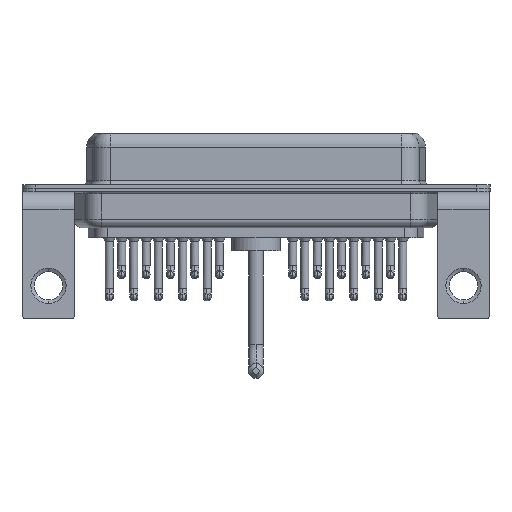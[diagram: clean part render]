
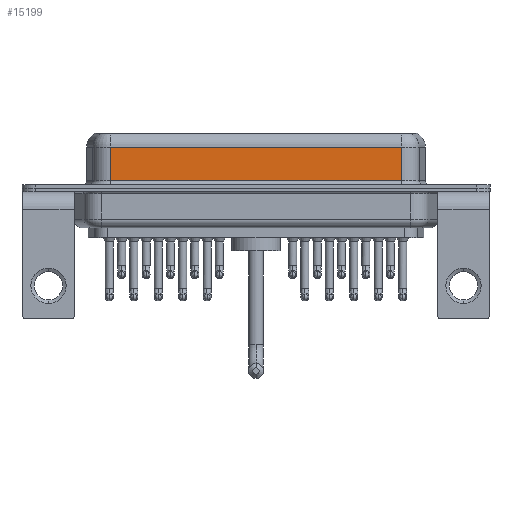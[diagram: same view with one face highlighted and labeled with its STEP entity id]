
A CAD part, front view. The second image highlights one B-rep face of the part: STEP entity #15199.
In plain terms, the highlighted planar face has unit normal (0, -1, 0).
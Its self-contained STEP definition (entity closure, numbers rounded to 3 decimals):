
#224 = DIRECTION ( 'NONE',  ( 0., 0., -1. ) ) ;
#295 = EDGE_LOOP ( 'NONE', ( #20281, #18069, #9514, #14334 ) ) ;
#2162 = CARTESIAN_POINT ( 'NONE',  ( 40.037, -3.95, 6.4 ) ) ;
#2310 = CARTESIAN_POINT ( 'NONE',  ( 40.037, -3.95, 4.65 ) ) ;
#2515 = CARTESIAN_POINT ( 'NONE',  ( 40.037, -3.95, 4.65 ) ) ;
#3378 = VECTOR ( 'NONE', #14742, 1000. ) ;
#3466 = VERTEX_POINT ( 'NONE', #2515 ) ;
#3902 = CARTESIAN_POINT ( 'NONE',  ( 7.013, -3.95, 6.4 ) ) ;
#4205 = CARTESIAN_POINT ( 'NONE',  ( 7.013, -3.95, 0.9 ) ) ;
#5093 = VECTOR ( 'NONE', #5467, 1000. ) ;
#5361 = VECTOR ( 'NONE', #8399, 1000. ) ;
#5467 = DIRECTION ( 'NONE',  ( 0., 0., -1. ) ) ;
#5949 = FACE_OUTER_BOUND ( 'NONE', #295, .T. ) ;
#6619 = CARTESIAN_POINT ( 'NONE',  ( 40.037, -3.95, 0.9 ) ) ;
#7416 = LINE ( 'NONE', #2310, #3378 ) ;
#7701 = VERTEX_POINT ( 'NONE', #11020 ) ;
#8399 = DIRECTION ( 'NONE',  ( 1., 0., 0. ) ) ;
#8780 = LINE ( 'NONE', #14222, #11009 ) ;
#9302 = EDGE_CURVE ( 'NONE', #3466, #20092, #7416, .T. ) ;
#9390 = DIRECTION ( 'NONE',  ( 0., 1., 0. ) ) ;
#9514 = ORIENTED_EDGE ( 'NONE', *, *, #11217, .T. ) ;
#11009 = VECTOR ( 'NONE', #224, 1000. ) ;
#11020 = CARTESIAN_POINT ( 'NONE',  ( 40.037, -3.95, 0.9 ) ) ;
#11175 = DIRECTION ( 'NONE',  ( 0., 0., 1. ) ) ;
#11217 = EDGE_CURVE ( 'NONE', #20092, #21561, #12791, .T. ) ;
#12791 = LINE ( 'NONE', #3902, #5093 ) ;
#13318 = AXIS2_PLACEMENT_3D ( 'NONE', #2162, #9390, #11175 ) ;
#14222 = CARTESIAN_POINT ( 'NONE',  ( 40.037, -3.95, 6.4 ) ) ;
#14334 = ORIENTED_EDGE ( 'NONE', *, *, #19742, .T. ) ;
#14742 = DIRECTION ( 'NONE',  ( -1., 0., 0. ) ) ;
#14987 = CARTESIAN_POINT ( 'NONE',  ( 7.013, -3.95, 4.65 ) ) ;
#15199 = ADVANCED_FACE ( 'NONE', ( #5949 ), #20360, .F. ) ;
#17370 = LINE ( 'NONE', #6619, #5361 ) ;
#18069 = ORIENTED_EDGE ( 'NONE', *, *, #9302, .T. ) ;
#19454 = EDGE_CURVE ( 'NONE', #3466, #7701, #8780, .T. ) ;
#19742 = EDGE_CURVE ( 'NONE', #21561, #7701, #17370, .T. ) ;
#20092 = VERTEX_POINT ( 'NONE', #14987 ) ;
#20281 = ORIENTED_EDGE ( 'NONE', *, *, #19454, .F. ) ;
#20360 = PLANE ( 'NONE',  #13318 ) ;
#21561 = VERTEX_POINT ( 'NONE', #4205 ) ;
